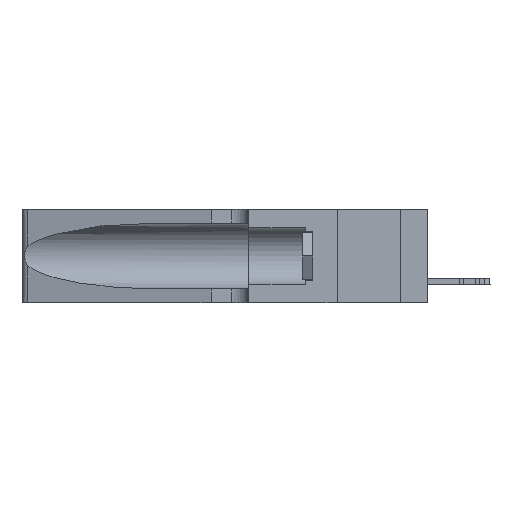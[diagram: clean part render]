
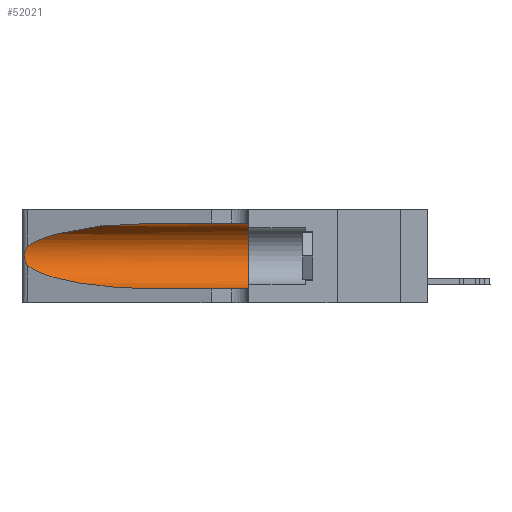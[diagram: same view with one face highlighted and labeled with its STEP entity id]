
A CAD part, left-side view. The second image highlights one B-rep face of the part: STEP entity #52021.
In plain terms, the highlighted cylindrical face has radius 3.308 mm (diameter 6.617 mm), a partial arc.
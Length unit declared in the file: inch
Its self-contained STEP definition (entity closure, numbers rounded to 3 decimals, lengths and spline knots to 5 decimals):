
#634 = AXIS2_PLACEMENT_3D ( 'NONE', #44604, #36007, #16037 ) ;
#1201 = LINE ( 'NONE', #9641, #17144 ) ;
#2420 = CARTESIAN_POINT ( 'NONE',  ( 0.25856, 1.23593, 0.16098 ) ) ;
#2736 = CARTESIAN_POINT ( 'NONE',  ( 0.2373, 1.15595, 0.28018 ) ) ;
#3258 = AXIS2_PLACEMENT_3D ( 'NONE', #44901, #8441, #28160 ) ;
#3797 = VERTEX_POINT ( 'NONE', #37795 ) ;
#4615 = CARTESIAN_POINT ( 'NONE',  ( 0.25487, 1.22718, 0.14631 ) ) ;
#4899 = DIRECTION ( 'NONE',  ( 0., -1., 0. ) ) ;
#5889 = CARTESIAN_POINT ( 'NONE',  ( 0.1305, 0.72297, 0.31525 ) ) ;
#6818 = CYLINDRICAL_SURFACE ( 'NONE', #634, 0.13025 ) ;
#6885 = CARTESIAN_POINT ( 'NONE',  ( 0.1305, 0.35, 0.05475 ) ) ;
#8236 = CARTESIAN_POINT ( 'NONE',  ( 0.1305, 0.72297, 0.05475 ) ) ;
#8441 = DIRECTION ( 'NONE',  ( 0., 1., 0. ) ) ;
#9231 = FACE_OUTER_BOUND ( 'NONE', #50093, .T. ) ;
#9641 = CARTESIAN_POINT ( 'NONE',  ( 0.1305, 1.61858, 0.31525 ) ) ;
#10227 = ORIENTED_EDGE ( 'NONE', *, *, #13705, .F. ) ;
#10228 = CARTESIAN_POINT ( 'NONE',  ( 0.25639, 1.23186, 0.15144 ) ) ;
#11007 = CARTESIAN_POINT ( 'NONE',  ( 0.25555, 1.22994, 0.2215 ) ) ;
#11134 = EDGE_CURVE ( 'NONE', #42092, #21674, #45481, .T. ) ;
#12904 = VERTEX_POINT ( 'NONE', #4615 ) ;
#13705 = EDGE_CURVE ( 'NONE', #3797, #21674, #49041, .T. ) ;
#14872 = CARTESIAN_POINT ( 'NONE',  ( 0.25487, 1.22718, 0.14631 ) ) ;
#15377 = EDGE_CURVE ( 'NONE', #51686, #12904, #28326, .T. ) ;
#16037 = DIRECTION ( 'NONE',  ( 0., 0., -1. ) ) ;
#16502 = VECTOR ( 'NONE', #4899, 39.37008 ) ;
#17144 = VECTOR ( 'NONE', #26204, 39.37008 ) ;
#17890 = VERTEX_POINT ( 'NONE', #34068 ) ;
#20371 = EDGE_CURVE ( 'NONE', #17890, #3797, #1201, .T. ) ;
#21674 = VERTEX_POINT ( 'NONE', #6885 ) ;
#22104 = ORIENTED_EDGE ( 'NONE', *, *, #15377, .T. ) ;
#22547 = CARTESIAN_POINT ( 'NONE',  ( 0.26075, 1.23896, 0.19203 ) ) ;
#22677 = CARTESIAN_POINT ( 'NONE',  ( 0.18966, 0.96281, 0.31525 ) ) ;
#22752 = CARTESIAN_POINT ( 'NONE',  ( 0.26018, 1.23835, 0.19895 ) ) ;
#23279 = CARTESIAN_POINT ( 'NONE',  ( 0.25487, 1.22718, 0.22369 ) ) ;
#23731 = ORIENTED_EDGE ( 'NONE', *, *, #28275, .T. ) ;
#25037 =( BOUNDED_CURVE ( )  B_SPLINE_CURVE ( 3, ( #5889, #22677, #2736, #35964 ),
 .UNSPECIFIED., .F., .F. ) 
 B_SPLINE_CURVE_WITH_KNOTS ( ( 4, 4 ),
 ( 1.5708, 2.84003 ),
 .UNSPECIFIED. ) 
 CURVE ( )  GEOMETRIC_REPRESENTATION_ITEM ( )  RATIONAL_B_SPLINE_CURVE ( ( 1., 0.87, 0.87, 1. ) ) 
 REPRESENTATION_ITEM ( '' )  );
#26204 = DIRECTION ( 'NONE',  ( 0., -1., 0. ) ) ;
#26415 = CARTESIAN_POINT ( 'NONE',  ( 0.26017, 1.23833, 0.17102 ) ) ;
#26829 = CARTESIAN_POINT ( 'NONE',  ( 0.2373, 1.15595, 0.08982 ) ) ;
#27788 = ORIENTED_EDGE ( 'NONE', *, *, #20371, .F. ) ;
#28091 = CARTESIAN_POINT ( 'NONE',  ( 0.1305, 1.61858, 0.05475 ) ) ;
#28160 = DIRECTION ( 'NONE',  ( 0., 0., 1. ) ) ;
#28275 = EDGE_CURVE ( 'NONE', #17890, #51686, #25037, .T. ) ;
#28326 = B_SPLINE_CURVE_WITH_KNOTS ( 'NONE', 3,
 ( #38810, #11007, #43266, #38615, #46782, #22752, #22547, #38995, #26415, #2420, #30633, #10228, #34738, #14872 ),
 .UNSPECIFIED., .F., .F.,
 ( 4, 2, 2, 2, 2, 2, 4 ),
 ( 0., 0.00027, 0.00053, 0.00107, 0.0016, 0.00187, 0.00214 ),
 .UNSPECIFIED. ) ;
#30468 = CARTESIAN_POINT ( 'NONE',  ( 0.18966, 0.96281, 0.05475 ) ) ;
#30633 = CARTESIAN_POINT ( 'NONE',  ( 0.25789, 1.23486, 0.15765 ) ) ;
#30670 = CARTESIAN_POINT ( 'NONE',  ( 0.1305, 0.72297, 0.05475 ) ) ;
#31203 = EDGE_CURVE ( 'NONE', #12904, #42092, #50283, .T. ) ;
#34068 = CARTESIAN_POINT ( 'NONE',  ( 0.1305, 0.72297, 0.31525 ) ) ;
#34738 = CARTESIAN_POINT ( 'NONE',  ( 0.25555, 1.22993, 0.14849 ) ) ;
#35155 = CARTESIAN_POINT ( 'NONE',  ( 0.25487, 1.22718, 0.14631 ) ) ;
#35964 = CARTESIAN_POINT ( 'NONE',  ( 0.25487, 1.22718, 0.22369 ) ) ;
#36007 = DIRECTION ( 'NONE',  ( 0., -1., 0. ) ) ;
#37795 = CARTESIAN_POINT ( 'NONE',  ( 0.1305, 0.35, 0.31525 ) ) ;
#38615 = CARTESIAN_POINT ( 'NONE',  ( 0.25787, 1.23484, 0.2124 ) ) ;
#38810 = CARTESIAN_POINT ( 'NONE',  ( 0.25487, 1.22718, 0.22369 ) ) ;
#38995 = CARTESIAN_POINT ( 'NONE',  ( 0.26075, 1.23896, 0.178 ) ) ;
#39832 = ORIENTED_EDGE ( 'NONE', *, *, #11134, .T. ) ;
#42092 = VERTEX_POINT ( 'NONE', #8236 ) ;
#43266 = CARTESIAN_POINT ( 'NONE',  ( 0.25639, 1.23184, 0.21858 ) ) ;
#43887 = ORIENTED_EDGE ( 'NONE', *, *, #31203, .T. ) ;
#44604 = CARTESIAN_POINT ( 'NONE',  ( 0.1305, 1.61858, 0.185 ) ) ;
#44901 = CARTESIAN_POINT ( 'NONE',  ( 0.1305, 0.35, 0.185 ) ) ;
#45481 = LINE ( 'NONE', #28091, #16502 ) ;
#46782 = CARTESIAN_POINT ( 'NONE',  ( 0.25854, 1.2359, 0.20912 ) ) ;
#49041 = CIRCLE ( 'NONE', #3258, 0.13025 ) ;
#50093 = EDGE_LOOP ( 'NONE', ( #23731, #22104, #43887, #39832, #10227, #27788 ) ) ;
#50283 =( BOUNDED_CURVE ( )  B_SPLINE_CURVE ( 3, ( #35155, #26829, #30468, #30670 ),
 .UNSPECIFIED., .F., .T. ) 
 B_SPLINE_CURVE_WITH_KNOTS ( ( 4, 4 ),
 ( 3.44316, 4.71239 ),
 .UNSPECIFIED. ) 
 CURVE ( )  GEOMETRIC_REPRESENTATION_ITEM ( )  RATIONAL_B_SPLINE_CURVE ( ( 1., 0.87, 0.87, 1. ) ) 
 REPRESENTATION_ITEM ( '' )  );
#51686 = VERTEX_POINT ( 'NONE', #23279 ) ;
#52021 = ADVANCED_FACE ( 'NONE', ( #9231 ), #6818, .F. ) ;
